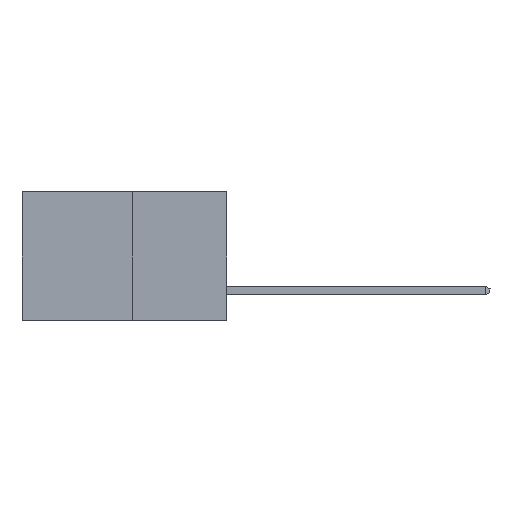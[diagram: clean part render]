
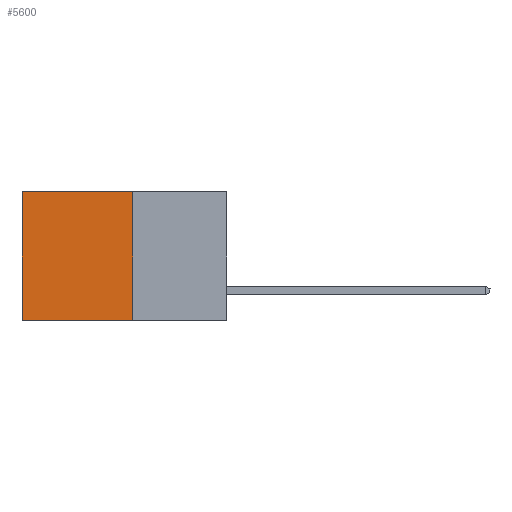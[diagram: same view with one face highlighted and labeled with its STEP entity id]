
A CAD part, left-side view. The second image highlights one B-rep face of the part: STEP entity #5600.
In plain terms, the highlighted planar face has unit normal (-1, 0, 0).
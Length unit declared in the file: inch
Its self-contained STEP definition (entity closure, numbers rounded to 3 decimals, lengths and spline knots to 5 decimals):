
#675 = CARTESIAN_POINT ( 'NONE',  ( 0.277, 0.27, -0.37 ) ) ;
#711 = VERTEX_POINT ( 'NONE', #12754 ) ;
#1220 = LINE ( 'NONE', #13406, #3843 ) ;
#1320 = CARTESIAN_POINT ( 'NONE',  ( 0.277, 0.27, 0. ) ) ;
#1465 = CARTESIAN_POINT ( 'NONE',  ( 0.277, 0.27, -0.37 ) ) ;
#1552 = EDGE_CURVE ( 'NONE', #8648, #11739, #4373, .T. ) ;
#1970 = AXIS2_PLACEMENT_3D ( 'NONE', #3631, #2076, #10721 ) ;
#2076 = DIRECTION ( 'NONE',  ( 1., 0., 0. ) ) ;
#2347 = DIRECTION ( 'NONE',  ( 0., 1., 0. ) ) ;
#3594 = VECTOR ( 'NONE', #7007, 39.37008 ) ;
#3631 = CARTESIAN_POINT ( 'NONE',  ( 0.277, 0.27, -0.37 ) ) ;
#3843 = VECTOR ( 'NONE', #6000, 39.37008 ) ;
#4133 = EDGE_CURVE ( 'NONE', #8648, #9012, #9393, .T. ) ;
#4373 = LINE ( 'NONE', #1465, #12579 ) ;
#4723 = VECTOR ( 'NONE', #2347, 39.37008 ) ;
#5423 = CARTESIAN_POINT ( 'NONE',  ( 0.277, 0.27, -0.37 ) ) ;
#5600 = ADVANCED_FACE ( 'NONE', ( #12678 ), #8855, .F. ) ;
#6000 = DIRECTION ( 'NONE',  ( 0., 0., -1. ) ) ;
#6216 = ORIENTED_EDGE ( 'NONE', *, *, #4133, .T. ) ;
#6266 = ORIENTED_EDGE ( 'NONE', *, *, #1552, .F. ) ;
#7007 = DIRECTION ( 'NONE',  ( 0., 1., 0. ) ) ;
#8613 = ORIENTED_EDGE ( 'NONE', *, *, #12908, .T. ) ;
#8648 = VERTEX_POINT ( 'NONE', #11754 ) ;
#8855 = PLANE ( 'NONE',  #1970 ) ;
#9012 = VERTEX_POINT ( 'NONE', #11725 ) ;
#9237 = ORIENTED_EDGE ( 'NONE', *, *, #12225, .F. ) ;
#9393 = LINE ( 'NONE', #1320, #3594 ) ;
#10523 = EDGE_LOOP ( 'NONE', ( #8613, #9237, #6266, #6216 ) ) ;
#10721 = DIRECTION ( 'NONE',  ( 0., 0., -1. ) ) ;
#11725 = CARTESIAN_POINT ( 'NONE',  ( 0.277, 0.59, 0. ) ) ;
#11739 = VERTEX_POINT ( 'NONE', #5423 ) ;
#11754 = CARTESIAN_POINT ( 'NONE',  ( 0.277, 0.27, 0. ) ) ;
#12225 = EDGE_CURVE ( 'NONE', #11739, #711, #13245, .T. ) ;
#12579 = VECTOR ( 'NONE', #12811, 39.37008 ) ;
#12678 = FACE_OUTER_BOUND ( 'NONE', #10523, .T. ) ;
#12754 = CARTESIAN_POINT ( 'NONE',  ( 0.277, 0.59, -0.37 ) ) ;
#12811 = DIRECTION ( 'NONE',  ( 0., 0., -1. ) ) ;
#12908 = EDGE_CURVE ( 'NONE', #9012, #711, #1220, .T. ) ;
#13245 = LINE ( 'NONE', #675, #4723 ) ;
#13406 = CARTESIAN_POINT ( 'NONE',  ( 0.277, 0.59, -0.37 ) ) ;
